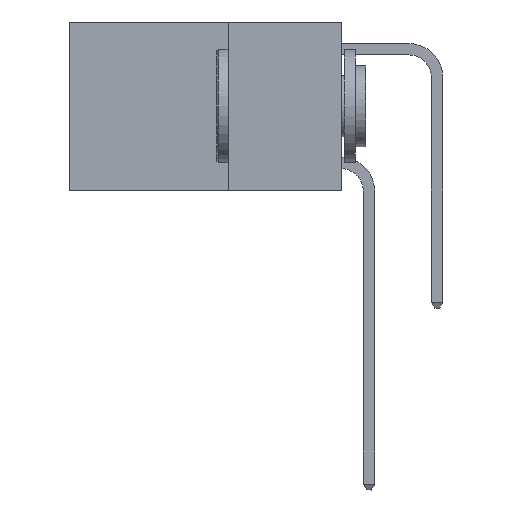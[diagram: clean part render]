
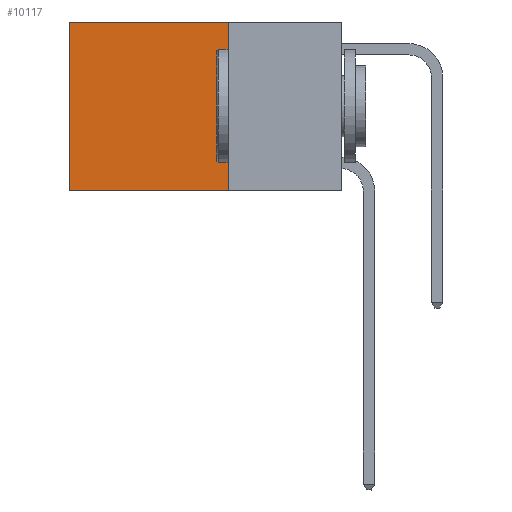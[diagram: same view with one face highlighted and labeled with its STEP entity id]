
A CAD part, left-side view. The second image highlights one B-rep face of the part: STEP entity #10117.
In plain terms, the highlighted planar face has unit normal (-1, 0, 0).
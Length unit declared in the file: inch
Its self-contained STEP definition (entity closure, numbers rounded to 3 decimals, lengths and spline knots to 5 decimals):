
#798 = EDGE_CURVE ( 'NONE', #4731, #7522, #13558, .T. ) ;
#1044 = PLANE ( 'NONE',  #4806 ) ;
#1171 = EDGE_CURVE ( 'NONE', #4727, #7522, #4912, .T. ) ;
#1480 = CARTESIAN_POINT ( 'NONE',  ( 0.2625, 0.25, -0.37 ) ) ;
#1564 = EDGE_CURVE ( 'NONE', #6731, #4731, #2430, .T. ) ;
#2197 = ORIENTED_EDGE ( 'NONE', *, *, #798, .T. ) ;
#2430 = LINE ( 'NONE', #4998, #5282 ) ;
#3518 = DIRECTION ( 'NONE',  ( 1., 0., 0. ) ) ;
#3822 = EDGE_CURVE ( 'NONE', #6731, #4727, #13661, .T. ) ;
#3931 = CARTESIAN_POINT ( 'NONE',  ( 0.2625, 0.6, 0. ) ) ;
#4046 = ORIENTED_EDGE ( 'NONE', *, *, #1564, .T. ) ;
#4416 = ORIENTED_EDGE ( 'NONE', *, *, #1171, .F. ) ;
#4727 = VERTEX_POINT ( 'NONE', #1480 ) ;
#4731 = VERTEX_POINT ( 'NONE', #3931 ) ;
#4806 = AXIS2_PLACEMENT_3D ( 'NONE', #9645, #3518, #12059 ) ;
#4912 = LINE ( 'NONE', #14472, #13947 ) ;
#4998 = CARTESIAN_POINT ( 'NONE',  ( 0.2625, 0.25, 0. ) ) ;
#5282 = VECTOR ( 'NONE', #5314, 39.37008 ) ;
#5314 = DIRECTION ( 'NONE',  ( 0., 1., 0. ) ) ;
#6372 = EDGE_LOOP ( 'NONE', ( #2197, #4416, #12935, #4046 ) ) ;
#6529 = CARTESIAN_POINT ( 'NONE',  ( 0.2625, 0.25, 0. ) ) ;
#6731 = VERTEX_POINT ( 'NONE', #8917 ) ;
#7102 = VECTOR ( 'NONE', #13944, 39.37008 ) ;
#7522 = VERTEX_POINT ( 'NONE', #7848 ) ;
#7815 = FACE_OUTER_BOUND ( 'NONE', #6372, .T. ) ;
#7848 = CARTESIAN_POINT ( 'NONE',  ( 0.2625, 0.6, -0.37 ) ) ;
#8409 = DIRECTION ( 'NONE',  ( 0., 0., -1. ) ) ;
#8917 = CARTESIAN_POINT ( 'NONE',  ( 0.2625, 0.25, 0. ) ) ;
#9645 = CARTESIAN_POINT ( 'NONE',  ( 0.2625, 0.25, 0. ) ) ;
#10117 = ADVANCED_FACE ( 'NONE', ( #7815 ), #1044, .F. ) ;
#12059 = DIRECTION ( 'NONE',  ( 0., 0., -1. ) ) ;
#12811 = VECTOR ( 'NONE', #8409, 39.37008 ) ;
#12907 = CARTESIAN_POINT ( 'NONE',  ( 0.2625, 0.6, 0. ) ) ;
#12935 = ORIENTED_EDGE ( 'NONE', *, *, #3822, .F. ) ;
#13558 = LINE ( 'NONE', #12907, #12811 ) ;
#13661 = LINE ( 'NONE', #6529, #7102 ) ;
#13944 = DIRECTION ( 'NONE',  ( 0., 0., -1. ) ) ;
#13947 = VECTOR ( 'NONE', #14546, 39.37008 ) ;
#14472 = CARTESIAN_POINT ( 'NONE',  ( 0.2625, 0.25, -0.37 ) ) ;
#14546 = DIRECTION ( 'NONE',  ( 0., 1., 0. ) ) ;
